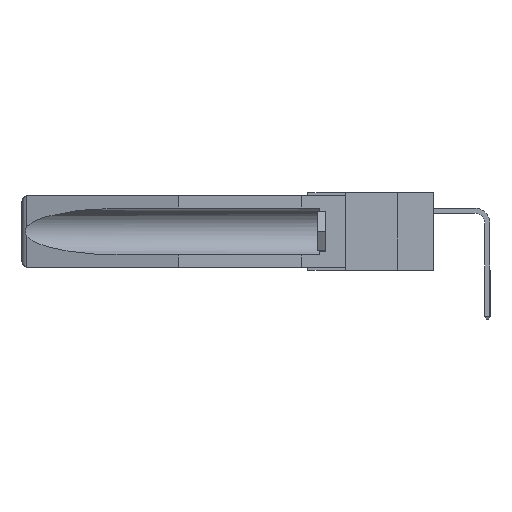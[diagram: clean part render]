
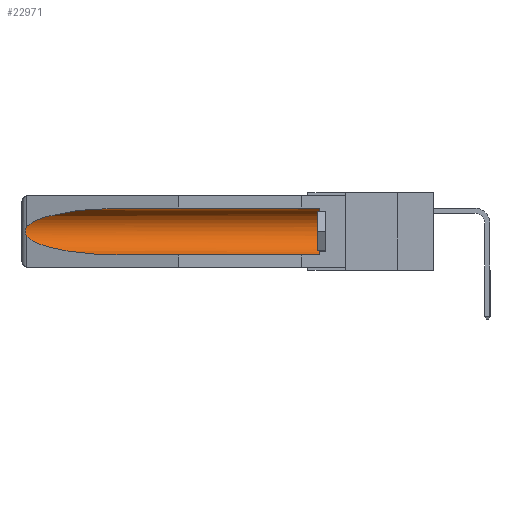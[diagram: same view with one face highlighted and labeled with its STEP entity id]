
A CAD part, left-side view. The second image highlights one B-rep face of the part: STEP entity #22971.
In plain terms, the highlighted cylindrical face has radius 2.857 mm (diameter 5.715 mm), a partial arc.
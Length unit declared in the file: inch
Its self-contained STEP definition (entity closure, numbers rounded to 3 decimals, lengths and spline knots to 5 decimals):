
#99 = CIRCLE ( 'NONE', #592, 0.1125 ) ;
#279 =( BOUNDED_CURVE ( )  B_SPLINE_CURVE ( 3, ( #8197, #19613, #4521, #2648 ),
 .UNSPECIFIED., .F., .F. ) 
 B_SPLINE_CURVE_WITH_KNOTS ( ( 4, 4 ),
 ( 0.1948, 1.5708 ),
 .UNSPECIFIED. ) 
 CURVE ( )  GEOMETRIC_REPRESENTATION_ITEM ( )  RATIONAL_B_SPLINE_CURVE ( ( 1., 0.848, 0.848, 1. ) ) 
 REPRESENTATION_ITEM ( '' )  );
#592 = AXIS2_PLACEMENT_3D ( 'NONE', #18120, #7867, #8309 ) ;
#927 = VERTEX_POINT ( 'NONE', #15021 ) ;
#1609 = CARTESIAN_POINT ( 'NONE',  ( 0.155, 1.07973, -0.284 ) ) ;
#2185 = VECTOR ( 'NONE', #8377, 39.37008 ) ;
#2601 = CARTESIAN_POINT ( 'NONE',  ( 0.26537, 1.52718, -0.14972 ) ) ;
#2648 = CARTESIAN_POINT ( 'NONE',  ( 0.155, 1.07973, -0.284 ) ) ;
#2733 = EDGE_CURVE ( 'NONE', #927, #20138, #14902, .T. ) ;
#2755 = CARTESIAN_POINT ( 'NONE',  ( 0.155, -0.30754, -0.284 ) ) ;
#4338 = EDGE_CURVE ( 'NONE', #20138, #9009, #7499, .T. ) ;
#4390 = CARTESIAN_POINT ( 'NONE',  ( 0.26654, 1.53092, -0.15636 ) ) ;
#4521 = CARTESIAN_POINT ( 'NONE',  ( 0.21114, 1.30732, -0.284 ) ) ;
#5773 = EDGE_CURVE ( 'NONE', #9009, #23794, #22874, .T. ) ;
#5892 = CARTESIAN_POINT ( 'NONE',  ( 0.21114, 1.30732, -0.059 ) ) ;
#6319 = CARTESIAN_POINT ( 'NONE',  ( 0.26597, 1.5296, -0.19026 ) ) ;
#6548 = DIRECTION ( 'NONE',  ( 0., 1., 0. ) ) ;
#7003 = DIRECTION ( 'NONE',  ( 0., 1., 0. ) ) ;
#7499 =( BOUNDED_CURVE ( )  B_SPLINE_CURVE ( 3, ( #13616, #5892, #23000, #15419 ),
 .UNSPECIFIED., .F., .F. ) 
 B_SPLINE_CURVE_WITH_KNOTS ( ( 4, 4 ),
 ( 4.71239, 6.08839 ),
 .UNSPECIFIED. ) 
 CURVE ( )  GEOMETRIC_REPRESENTATION_ITEM ( )  RATIONAL_B_SPLINE_CURVE ( ( 1., 0.848, 0.848, 1. ) ) 
 REPRESENTATION_ITEM ( '' )  );
#7867 = DIRECTION ( 'NONE',  ( 0., -1., 0. ) ) ;
#8197 = CARTESIAN_POINT ( 'NONE',  ( 0.26537, 1.52718, -0.19328 ) ) ;
#8305 = ORIENTED_EDGE ( 'NONE', *, *, #22023, .F. ) ;
#8309 = DIRECTION ( 'NONE',  ( 0., 0., 1. ) ) ;
#8314 = EDGE_CURVE ( 'NONE', #23794, #18479, #279, .T. ) ;
#8377 = DIRECTION ( 'NONE',  ( 0., 1., 0. ) ) ;
#9009 = VERTEX_POINT ( 'NONE', #18097 ) ;
#9850 = VECTOR ( 'NONE', #7003, 39.37008 ) ;
#9854 = CARTESIAN_POINT ( 'NONE',  ( 0.26537, 1.52718, -0.19328 ) ) ;
#10039 = CARTESIAN_POINT ( 'NONE',  ( 0.2675, 1.53308, -0.16763 ) ) ;
#10115 = CARTESIAN_POINT ( 'NONE',  ( 0.2673, 1.53269, -0.17917 ) ) ;
#10205 = AXIS2_PLACEMENT_3D ( 'NONE', #15903, #6548, #19808 ) ;
#10286 = CARTESIAN_POINT ( 'NONE',  ( 0.26597, 1.52961, -0.15275 ) ) ;
#10891 = ORIENTED_EDGE ( 'NONE', *, *, #8314, .T. ) ;
#11237 = EDGE_CURVE ( 'NONE', #16560, #927, #99, .T. ) ;
#11975 = CARTESIAN_POINT ( 'NONE',  ( 0.2675, 1.53308, -0.17534 ) ) ;
#12085 = ORIENTED_EDGE ( 'NONE', *, *, #2733, .T. ) ;
#12708 = ORIENTED_EDGE ( 'NONE', *, *, #11237, .T. ) ;
#13616 = CARTESIAN_POINT ( 'NONE',  ( 0.155, 1.07973, -0.059 ) ) ;
#14902 = LINE ( 'NONE', #18429, #9850 ) ;
#15021 = CARTESIAN_POINT ( 'NONE',  ( 0.155, 0.126, -0.059 ) ) ;
#15419 = CARTESIAN_POINT ( 'NONE',  ( 0.26537, 1.52718, -0.14972 ) ) ;
#15903 = CARTESIAN_POINT ( 'NONE',  ( 0.155, -0.30754, -0.1715 ) ) ;
#16076 = EDGE_LOOP ( 'NONE', ( #24352, #19239, #10891, #8305, #12708, #12085 ) ) ;
#16231 = FACE_OUTER_BOUND ( 'NONE', #16076, .T. ) ;
#16560 = VERTEX_POINT ( 'NONE', #24306 ) ;
#17685 = CARTESIAN_POINT ( 'NONE',  ( 0.26655, 1.53094, -0.18657 ) ) ;
#17756 = CARTESIAN_POINT ( 'NONE',  ( 0.26537, 1.52718, -0.19328 ) ) ;
#18097 = CARTESIAN_POINT ( 'NONE',  ( 0.26537, 1.52718, -0.14972 ) ) ;
#18120 = CARTESIAN_POINT ( 'NONE',  ( 0.155, 0.126, -0.1715 ) ) ;
#18429 = CARTESIAN_POINT ( 'NONE',  ( 0.155, -0.30754, -0.059 ) ) ;
#18479 = VERTEX_POINT ( 'NONE', #1609 ) ;
#18892 = CYLINDRICAL_SURFACE ( 'NONE', #10205, 0.1125 ) ;
#19145 = LINE ( 'NONE', #2755, #2185 ) ;
#19239 = ORIENTED_EDGE ( 'NONE', *, *, #5773, .T. ) ;
#19613 = CARTESIAN_POINT ( 'NONE',  ( 0.25451, 1.48313, -0.24835 ) ) ;
#19739 = CARTESIAN_POINT ( 'NONE',  ( 0.2673, 1.5327, -0.16383 ) ) ;
#19808 = DIRECTION ( 'NONE',  ( 0., 0., 1. ) ) ;
#20138 = VERTEX_POINT ( 'NONE', #20968 ) ;
#20968 = CARTESIAN_POINT ( 'NONE',  ( 0.155, 1.07973, -0.059 ) ) ;
#22023 = EDGE_CURVE ( 'NONE', #16560, #18479, #19145, .T. ) ;
#22874 = B_SPLINE_CURVE_WITH_KNOTS ( 'NONE', 3,
 ( #2601, #10286, #4390, #19739, #10039, #11975, #10115, #17685, #6319, #17756 ),
 .UNSPECIFIED., .F., .F.,
 ( 4, 2, 2, 2, 4 ),
 ( 0., 0.00029, 0.00058, 0.00087, 0.00117 ),
 .UNSPECIFIED. ) ;
#22971 = ADVANCED_FACE ( 'NONE', ( #16231 ), #18892, .F. ) ;
#23000 = CARTESIAN_POINT ( 'NONE',  ( 0.25451, 1.48313, -0.09465 ) ) ;
#23794 = VERTEX_POINT ( 'NONE', #9854 ) ;
#24306 = CARTESIAN_POINT ( 'NONE',  ( 0.155, 0.126, -0.284 ) ) ;
#24352 = ORIENTED_EDGE ( 'NONE', *, *, #4338, .T. ) ;
